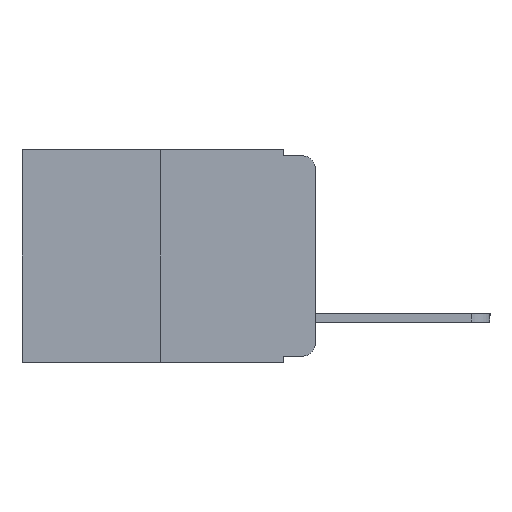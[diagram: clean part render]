
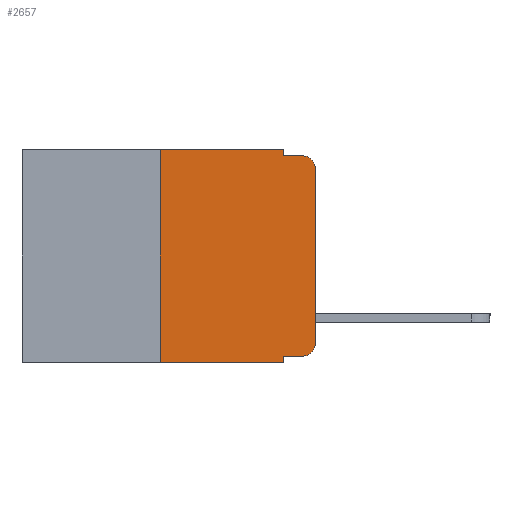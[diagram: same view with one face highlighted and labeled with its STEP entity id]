
A CAD part, left-side view. The second image highlights one B-rep face of the part: STEP entity #2657.
In plain terms, the highlighted planar face has unit normal (-1, 0, 0).
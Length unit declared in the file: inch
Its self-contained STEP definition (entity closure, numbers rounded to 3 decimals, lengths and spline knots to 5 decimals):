
#456 = VERTEX_POINT ( 'NONE', #15014 ) ;
#1244 = DIRECTION ( 'NONE',  ( -1., 0., 0. ) ) ;
#1448 = EDGE_CURVE ( 'NONE', #15839, #13742, #11682, .T. ) ;
#1487 = ORIENTED_EDGE ( 'NONE', *, *, #18616, .F. ) ;
#1505 = LINE ( 'NONE', #18287, #16615 ) ;
#1562 = VECTOR ( 'NONE', #12645, 39.37008 ) ;
#1698 = VERTEX_POINT ( 'NONE', #5607 ) ;
#2098 = VERTEX_POINT ( 'NONE', #16461 ) ;
#2102 = LINE ( 'NONE', #18112, #10274 ) ;
#2214 = ORIENTED_EDGE ( 'NONE', *, *, #10847, .T. ) ;
#2302 = DIRECTION ( 'NONE',  ( 0., -1., 0. ) ) ;
#2404 = ORIENTED_EDGE ( 'NONE', *, *, #16678, .F. ) ;
#2474 = DIRECTION ( 'NONE',  ( 0., 0., 1. ) ) ;
#2642 = CARTESIAN_POINT ( 'NONE',  ( 0., 0.473, 0. ) ) ;
#2657 = ADVANCED_FACE ( 'NONE', ( #11233 ), #7687, .F. ) ;
#2839 = CARTESIAN_POINT ( 'NONE',  ( 0., 0.25, -0.343 ) ) ;
#2888 = CARTESIAN_POINT ( 'NONE',  ( 0., 0.25, 0. ) ) ;
#3082 = VERTEX_POINT ( 'NONE', #11865 ) ;
#3617 = ORIENTED_EDGE ( 'NONE', *, *, #16320, .T. ) ;
#3978 = VECTOR ( 'NONE', #2474, 39.37008 ) ;
#4330 = VECTOR ( 'NONE', #2302, 39.37008 ) ;
#4352 = DIRECTION ( 'NONE',  ( 0., -1., 0. ) ) ;
#4612 = CARTESIAN_POINT ( 'NONE',  ( 0., 0.051, -0.343 ) ) ;
#4801 = EDGE_CURVE ( 'NONE', #8447, #2098, #5896, .T. ) ;
#5108 = DIRECTION ( 'NONE',  ( 0., 0., -1. ) ) ;
#5505 = ORIENTED_EDGE ( 'NONE', *, *, #15329, .T. ) ;
#5607 = CARTESIAN_POINT ( 'NONE',  ( 0., 0., -0.03 ) ) ;
#5720 = VERTEX_POINT ( 'NONE', #2839 ) ;
#5896 = LINE ( 'NONE', #12771, #1562 ) ;
#6396 = CIRCLE ( 'NONE', #18356, 0.02 ) ;
#6493 = ORIENTED_EDGE ( 'NONE', *, *, #1448, .F. ) ;
#6773 = VECTOR ( 'NONE', #15108, 39.37008 ) ;
#7359 = VECTOR ( 'NONE', #4352, 39.37008 ) ;
#7552 = EDGE_CURVE ( 'NONE', #456, #3082, #11165, .T. ) ;
#7602 = CIRCLE ( 'NONE', #15999, 0.02 ) ;
#7679 = EDGE_CURVE ( 'NONE', #2098, #12424, #6396, .T. ) ;
#7687 = PLANE ( 'NONE',  #8242 ) ;
#7747 = DIRECTION ( 'NONE',  ( -1., 0., 0. ) ) ;
#7957 = DIRECTION ( 'NONE',  ( 0., 0., -1. ) ) ;
#8144 = ORIENTED_EDGE ( 'NONE', *, *, #7552, .F. ) ;
#8242 = AXIS2_PLACEMENT_3D ( 'NONE', #2642, #17868, #15825 ) ;
#8447 = VERTEX_POINT ( 'NONE', #19349 ) ;
#8511 = LINE ( 'NONE', #11479, #3978 ) ;
#9426 = EDGE_LOOP ( 'NONE', ( #3617, #5505, #8144, #14924, #6493, #1487, #2214, #2404, #13881, #17732 ) ) ;
#10274 = VECTOR ( 'NONE', #7957, 39.37008 ) ;
#10547 = CARTESIAN_POINT ( 'NONE',  ( 0., 0.02, -0.313 ) ) ;
#10637 = LINE ( 'NONE', #12113, #6773 ) ;
#10847 = EDGE_CURVE ( 'NONE', #5720, #15898, #1505, .T. ) ;
#11165 = LINE ( 'NONE', #16106, #7359 ) ;
#11233 = FACE_OUTER_BOUND ( 'NONE', #9426, .T. ) ;
#11479 = CARTESIAN_POINT ( 'NONE',  ( 0., 0., 0. ) ) ;
#11682 = LINE ( 'NONE', #15127, #4330 ) ;
#11865 = CARTESIAN_POINT ( 'NONE',  ( 0., 0.02, -0.01 ) ) ;
#11914 = DIRECTION ( 'NONE',  ( 0., 0., -1. ) ) ;
#12103 = CARTESIAN_POINT ( 'NONE',  ( 0., 0.051, 0. ) ) ;
#12113 = CARTESIAN_POINT ( 'NONE',  ( 0., 0.25, 0. ) ) ;
#12424 = VERTEX_POINT ( 'NONE', #13302 ) ;
#12645 = DIRECTION ( 'NONE',  ( 0., -1., 0. ) ) ;
#12771 = CARTESIAN_POINT ( 'NONE',  ( 0., 0.051, -0.333 ) ) ;
#13302 = CARTESIAN_POINT ( 'NONE',  ( 0., 0., -0.313 ) ) ;
#13742 = VERTEX_POINT ( 'NONE', #12103 ) ;
#13881 = ORIENTED_EDGE ( 'NONE', *, *, #4801, .T. ) ;
#14924 = ORIENTED_EDGE ( 'NONE', *, *, #19556, .F. ) ;
#15014 = CARTESIAN_POINT ( 'NONE',  ( 0., 0.051, -0.01 ) ) ;
#15108 = DIRECTION ( 'NONE',  ( 0., 0., 1. ) ) ;
#15127 = CARTESIAN_POINT ( 'NONE',  ( 0., 0.473, 0. ) ) ;
#15329 = EDGE_CURVE ( 'NONE', #1698, #3082, #7602, .T. ) ;
#15825 = DIRECTION ( 'NONE',  ( 0., 0., -1. ) ) ;
#15839 = VERTEX_POINT ( 'NONE', #2888 ) ;
#15898 = VERTEX_POINT ( 'NONE', #4612 ) ;
#15999 = AXIS2_PLACEMENT_3D ( 'NONE', #16434, #7747, #17900 ) ;
#16106 = CARTESIAN_POINT ( 'NONE',  ( 0., 0.051, -0.01 ) ) ;
#16320 = EDGE_CURVE ( 'NONE', #12424, #1698, #8511, .T. ) ;
#16325 = VECTOR ( 'NONE', #5108, 39.37008 ) ;
#16434 = CARTESIAN_POINT ( 'NONE',  ( 0., 0.02, -0.03 ) ) ;
#16461 = CARTESIAN_POINT ( 'NONE',  ( 0., 0.02, -0.333 ) ) ;
#16615 = VECTOR ( 'NONE', #19683, 39.37008 ) ;
#16678 = EDGE_CURVE ( 'NONE', #8447, #15898, #2102, .T. ) ;
#17732 = ORIENTED_EDGE ( 'NONE', *, *, #7679, .T. ) ;
#17868 = DIRECTION ( 'NONE',  ( 1., 0., 0. ) ) ;
#17900 = DIRECTION ( 'NONE',  ( 0., 0., -1. ) ) ;
#18112 = CARTESIAN_POINT ( 'NONE',  ( 0., 0.051, 0. ) ) ;
#18287 = CARTESIAN_POINT ( 'NONE',  ( 0., 0.473, -0.343 ) ) ;
#18356 = AXIS2_PLACEMENT_3D ( 'NONE', #10547, #1244, #11914 ) ;
#18420 = CARTESIAN_POINT ( 'NONE',  ( 0., 0.051, 0. ) ) ;
#18616 = EDGE_CURVE ( 'NONE', #5720, #15839, #10637, .T. ) ;
#19349 = CARTESIAN_POINT ( 'NONE',  ( 0., 0.051, -0.333 ) ) ;
#19556 = EDGE_CURVE ( 'NONE', #13742, #456, #19681, .T. ) ;
#19681 = LINE ( 'NONE', #18420, #16325 ) ;
#19683 = DIRECTION ( 'NONE',  ( 0., -1., 0. ) ) ;
